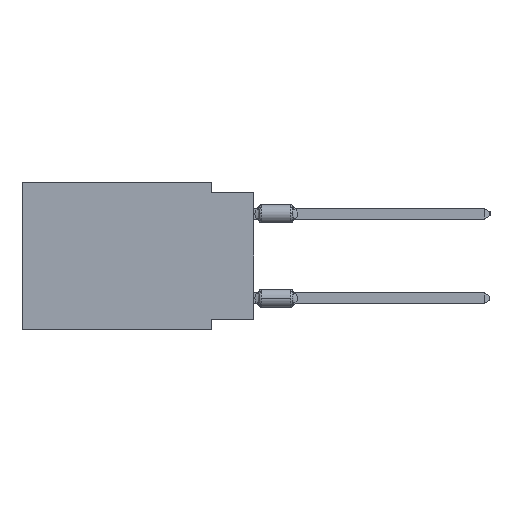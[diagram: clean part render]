
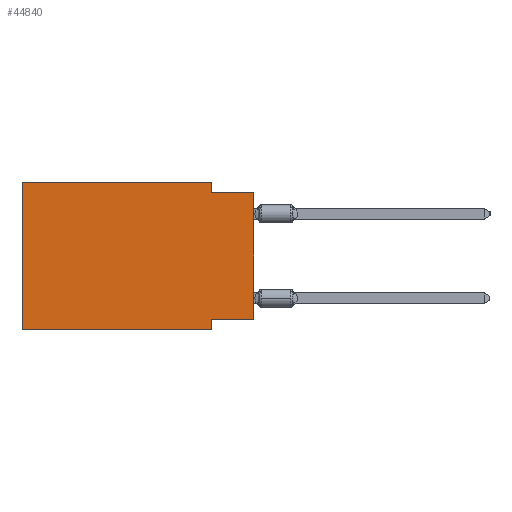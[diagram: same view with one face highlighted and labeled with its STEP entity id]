
A CAD part, left-side view. The second image highlights one B-rep face of the part: STEP entity #44840.
In plain terms, the highlighted planar face has unit normal (-1, 0, 0).
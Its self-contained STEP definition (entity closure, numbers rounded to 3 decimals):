
#17 = LINE ( 'NONE', #34399, #3279 ) ;
#1366 = LINE ( 'NONE', #32907, #50706 ) ;
#2027 = DIRECTION ( 'NONE',  ( 0., 0., 1. ) ) ;
#3279 = VECTOR ( 'NONE', #12510, 1000. ) ;
#3947 = EDGE_CURVE ( 'NONE', #23241, #47887, #15289, .T. ) ;
#4955 = EDGE_CURVE ( 'NONE', #23928, #49339, #6489, .T. ) ;
#6489 = LINE ( 'NONE', #11315, #22735 ) ;
#7613 = CARTESIAN_POINT ( 'NONE',  ( 0., 0., -0.635 ) ) ;
#7686 = VECTOR ( 'NONE', #7890, 1000. ) ;
#7723 = DIRECTION ( 'NONE',  ( 0., 0., -1. ) ) ;
#7890 = DIRECTION ( 'NONE',  ( 0., -1., 0. ) ) ;
#8352 = EDGE_LOOP ( 'NONE', ( #55584, #24091, #40504, #26983, #21097, #48506, #31778, #21093 ) ) ;
#9251 = CARTESIAN_POINT ( 'NONE',  ( 0., 0., -0.635 ) ) ;
#11315 = CARTESIAN_POINT ( 'NONE',  ( 0., 13.97, -8.89 ) ) ;
#12084 = VECTOR ( 'NONE', #2027, 1000. ) ;
#12510 = DIRECTION ( 'NONE',  ( 0., 0., -1. ) ) ;
#12637 = DIRECTION ( 'NONE',  ( 0., -1., 0. ) ) ;
#13015 = CARTESIAN_POINT ( 'NONE',  ( 0., 0., -8.255 ) ) ;
#13678 = CARTESIAN_POINT ( 'NONE',  ( 0., 2.54, -0.635 ) ) ;
#13864 = EDGE_CURVE ( 'NONE', #23516, #49339, #17, .T. ) ;
#14442 = CARTESIAN_POINT ( 'NONE',  ( 0., 2.54, 0. ) ) ;
#15111 = LINE ( 'NONE', #53810, #12084 ) ;
#15289 = LINE ( 'NONE', #14442, #47558 ) ;
#17023 = CARTESIAN_POINT ( 'NONE',  ( 0., 2.54, 0. ) ) ;
#18651 = EDGE_CURVE ( 'NONE', #43090, #23241, #33970, .T. ) ;
#20142 = LINE ( 'NONE', #7613, #7686 ) ;
#20676 = EDGE_CURVE ( 'NONE', #23928, #43090, #15111, .T. ) ;
#21093 = ORIENTED_EDGE ( 'NONE', *, *, #28668, .F. ) ;
#21097 = ORIENTED_EDGE ( 'NONE', *, *, #20676, .F. ) ;
#22425 = VERTEX_POINT ( 'NONE', #9251 ) ;
#22735 = VECTOR ( 'NONE', #24376, 1000. ) ;
#22824 = CARTESIAN_POINT ( 'NONE',  ( 0., 0., -8.255 ) ) ;
#23166 = CARTESIAN_POINT ( 'NONE',  ( 0., 13.97, -8.89 ) ) ;
#23241 = VERTEX_POINT ( 'NONE', #17023 ) ;
#23516 = VERTEX_POINT ( 'NONE', #27509 ) ;
#23928 = VERTEX_POINT ( 'NONE', #23166 ) ;
#24091 = ORIENTED_EDGE ( 'NONE', *, *, #34077, .F. ) ;
#24376 = DIRECTION ( 'NONE',  ( 0., -1., 0. ) ) ;
#26553 = CARTESIAN_POINT ( 'NONE',  ( 0., 2.54, -8.89 ) ) ;
#26983 = ORIENTED_EDGE ( 'NONE', *, *, #18651, .F. ) ;
#27509 = CARTESIAN_POINT ( 'NONE',  ( 0., 2.54, -8.255 ) ) ;
#28374 = DIRECTION ( 'NONE',  ( 0., 0., -1. ) ) ;
#28430 = VECTOR ( 'NONE', #12637, 1000. ) ;
#28668 = EDGE_CURVE ( 'NONE', #52236, #23516, #32460, .T. ) ;
#31778 = ORIENTED_EDGE ( 'NONE', *, *, #13864, .F. ) ;
#32460 = LINE ( 'NONE', #22824, #47064 ) ;
#32618 = DIRECTION ( 'NONE',  ( 0., 0., 1. ) ) ;
#32907 = CARTESIAN_POINT ( 'NONE',  ( 0., 0., 0. ) ) ;
#33970 = LINE ( 'NONE', #55906, #28430 ) ;
#34077 = EDGE_CURVE ( 'NONE', #47887, #22425, #20142, .T. ) ;
#34399 = CARTESIAN_POINT ( 'NONE',  ( 0., 2.54, -8.89 ) ) ;
#34429 = CARTESIAN_POINT ( 'NONE',  ( 0., 13.97, 0. ) ) ;
#36641 = AXIS2_PLACEMENT_3D ( 'NONE', #34429, #55527, #7723 ) ;
#38386 = CARTESIAN_POINT ( 'NONE',  ( 0., 13.97, 0. ) ) ;
#38716 = PLANE ( 'NONE',  #36641 ) ;
#38987 = FACE_OUTER_BOUND ( 'NONE', #8352, .T. ) ;
#40504 = ORIENTED_EDGE ( 'NONE', *, *, #3947, .F. ) ;
#43090 = VERTEX_POINT ( 'NONE', #38386 ) ;
#44840 = ADVANCED_FACE ( 'NONE', ( #38987 ), #38716, .F. ) ;
#47064 = VECTOR ( 'NONE', #53825, 1000. ) ;
#47558 = VECTOR ( 'NONE', #28374, 1000. ) ;
#47887 = VERTEX_POINT ( 'NONE', #13678 ) ;
#48506 = ORIENTED_EDGE ( 'NONE', *, *, #4955, .T. ) ;
#48720 = EDGE_CURVE ( 'NONE', #52236, #22425, #1366, .T. ) ;
#49339 = VERTEX_POINT ( 'NONE', #26553 ) ;
#50706 = VECTOR ( 'NONE', #32618, 1000. ) ;
#52236 = VERTEX_POINT ( 'NONE', #13015 ) ;
#53810 = CARTESIAN_POINT ( 'NONE',  ( 0., 13.97, 0. ) ) ;
#53825 = DIRECTION ( 'NONE',  ( 0., 1., 0. ) ) ;
#55527 = DIRECTION ( 'NONE',  ( 1., 0., 0. ) ) ;
#55584 = ORIENTED_EDGE ( 'NONE', *, *, #48720, .T. ) ;
#55906 = CARTESIAN_POINT ( 'NONE',  ( 0., 13.97, 0. ) ) ;
